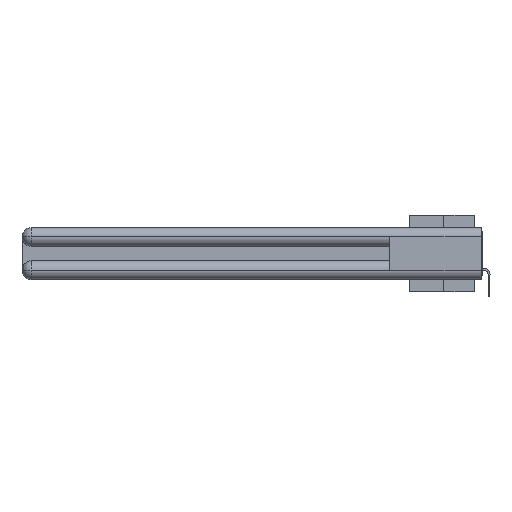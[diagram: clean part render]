
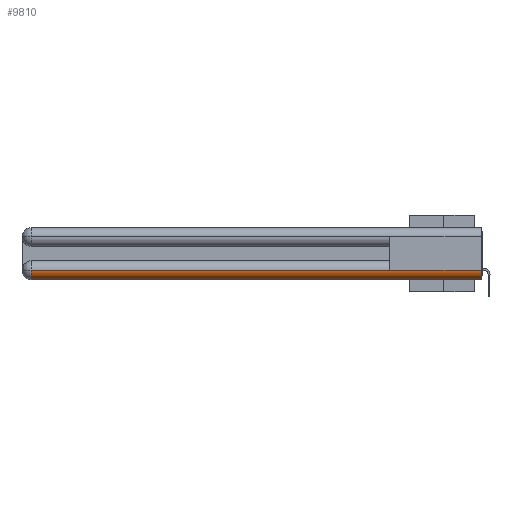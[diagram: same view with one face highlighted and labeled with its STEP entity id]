
A CAD part, left-side view. The second image highlights one B-rep face of the part: STEP entity #9810.
In plain terms, the highlighted cylindrical face has radius 1.562 mm (diameter 3.124 mm), a partial arc.
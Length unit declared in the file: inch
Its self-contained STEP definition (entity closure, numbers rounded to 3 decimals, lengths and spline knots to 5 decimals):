
#976 = EDGE_LOOP ( 'NONE', ( #32349, #1308, #23694, #22947, #27319 ) ) ;
#1151 = CARTESIAN_POINT ( 'NONE',  ( 0., 2.94, -0.2785 ) ) ;
#1281 = EDGE_CURVE ( 'NONE', #6345, #11934, #23226, .T. ) ;
#1308 = ORIENTED_EDGE ( 'NONE', *, *, #4560, .T. ) ;
#1440 = CARTESIAN_POINT ( 'NONE',  ( 0., 0.6, -0.2785 ) ) ;
#4225 = DIRECTION ( 'NONE',  ( 0., 1., 0. ) ) ;
#4431 = CARTESIAN_POINT ( 'NONE',  ( 0., 0., -0.2785 ) ) ;
#4560 = EDGE_CURVE ( 'NONE', #25950, #7108, #18533, .T. ) ;
#5373 = CARTESIAN_POINT ( 'NONE',  ( 0., 0., -0.2785 ) ) ;
#5622 = CARTESIAN_POINT ( 'NONE',  ( 0.0615, 2.94, -0.34 ) ) ;
#6345 = VERTEX_POINT ( 'NONE', #1440 ) ;
#6580 = VECTOR ( 'NONE', #22588, 39.37008 ) ;
#7108 = VERTEX_POINT ( 'NONE', #5622 ) ;
#7129 = LINE ( 'NONE', #27662, #11623 ) ;
#9053 = DIRECTION ( 'NONE',  ( 0., 0., -1. ) ) ;
#9810 = ADVANCED_FACE ( 'NONE', ( #31960 ), #30338, .T. ) ;
#9949 = CARTESIAN_POINT ( 'NONE',  ( 0.0615, 2.94, -0.2785 ) ) ;
#11290 = VERTEX_POINT ( 'NONE', #19980 ) ;
#11310 = EDGE_CURVE ( 'NONE', #11290, #7108, #7129, .T. ) ;
#11328 = CARTESIAN_POINT ( 'NONE',  ( 0.0615, 0., -0.2785 ) ) ;
#11623 = VECTOR ( 'NONE', #4225, 39.37008 ) ;
#11934 = VERTEX_POINT ( 'NONE', #5373 ) ;
#13437 = LINE ( 'NONE', #4431, #6580 ) ;
#13919 = DIRECTION ( 'NONE',  ( 0., -1., 0. ) ) ;
#16274 = VECTOR ( 'NONE', #18081, 39.37008 ) ;
#16831 = DIRECTION ( 'NONE',  ( 0., -1., 0. ) ) ;
#18081 = DIRECTION ( 'NONE',  ( 0., -1., 0. ) ) ;
#18533 = CIRCLE ( 'NONE', #26622, 0.0615 ) ;
#19980 = CARTESIAN_POINT ( 'NONE',  ( 0.0615, 0., -0.34 ) ) ;
#21633 = CARTESIAN_POINT ( 'NONE',  ( 0.0615, 0., -0.2785 ) ) ;
#22588 = DIRECTION ( 'NONE',  ( 0., 1., 0. ) ) ;
#22947 = ORIENTED_EDGE ( 'NONE', *, *, #25212, .F. ) ;
#23226 = LINE ( 'NONE', #33510, #16274 ) ;
#23694 = ORIENTED_EDGE ( 'NONE', *, *, #11310, .F. ) ;
#23803 = CIRCLE ( 'NONE', #26504, 0.0615 ) ;
#24396 = AXIS2_PLACEMENT_3D ( 'NONE', #21633, #16831, #9053 ) ;
#25212 = EDGE_CURVE ( 'NONE', #11934, #11290, #23803, .T. ) ;
#25950 = VERTEX_POINT ( 'NONE', #1151 ) ;
#26504 = AXIS2_PLACEMENT_3D ( 'NONE', #11328, #13919, #27055 ) ;
#26622 = AXIS2_PLACEMENT_3D ( 'NONE', #9949, #30550, #30874 ) ;
#27055 = DIRECTION ( 'NONE',  ( 1., 0., 0. ) ) ;
#27319 = ORIENTED_EDGE ( 'NONE', *, *, #1281, .F. ) ;
#27662 = CARTESIAN_POINT ( 'NONE',  ( 0.0615, 0., -0.34 ) ) ;
#30091 = EDGE_CURVE ( 'NONE', #6345, #25950, #13437, .T. ) ;
#30338 = CYLINDRICAL_SURFACE ( 'NONE', #24396, 0.0615 ) ;
#30550 = DIRECTION ( 'NONE',  ( 0., -1., 0. ) ) ;
#30874 = DIRECTION ( 'NONE',  ( 0., 0., 1. ) ) ;
#31960 = FACE_OUTER_BOUND ( 'NONE', #976, .T. ) ;
#32349 = ORIENTED_EDGE ( 'NONE', *, *, #30091, .T. ) ;
#33510 = CARTESIAN_POINT ( 'NONE',  ( 0., 0., -0.2785 ) ) ;
